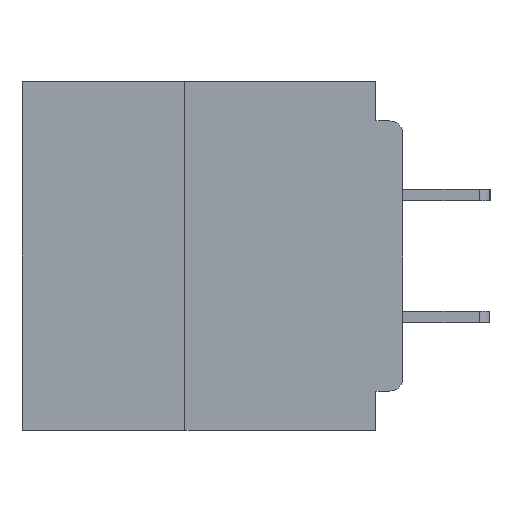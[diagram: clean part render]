
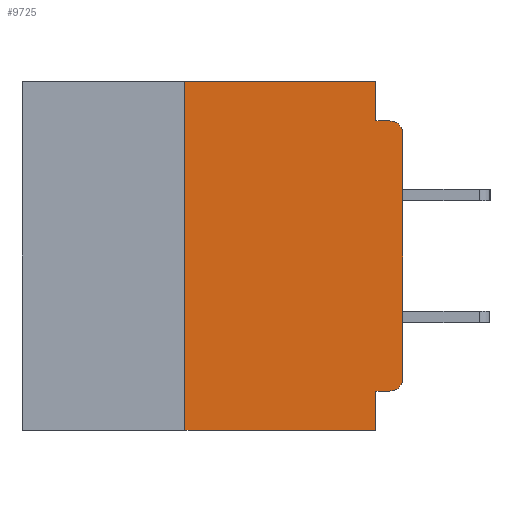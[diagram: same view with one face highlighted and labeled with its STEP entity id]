
A CAD part, left-side view. The second image highlights one B-rep face of the part: STEP entity #9725.
In plain terms, the highlighted planar face has unit normal (-1, 0, 0).
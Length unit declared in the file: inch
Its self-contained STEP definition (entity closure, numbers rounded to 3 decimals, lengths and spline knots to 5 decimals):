
#355 = EDGE_CURVE ( 'NONE', #34685, #10044, #22795, .T. ) ;
#2576 = DIRECTION ( 'NONE',  ( 0., 1., 0. ) ) ;
#2628 = CARTESIAN_POINT ( 'NONE',  ( 0., 0., -0.045 ) ) ;
#3607 = EDGE_CURVE ( 'NONE', #11408, #34685, #57170, .T. ) ;
#4150 = VECTOR ( 'NONE', #14899, 39.37008 ) ;
#4229 = ORIENTED_EDGE ( 'NONE', *, *, #5340, .T. ) ;
#5340 = EDGE_CURVE ( 'NONE', #44984, #27405, #8590, .T. ) ;
#5851 = CARTESIAN_POINT ( 'NONE',  ( 0., 0.015, -0.355 ) ) ;
#6154 = VERTEX_POINT ( 'NONE', #36166 ) ;
#6261 = DIRECTION ( 'NONE',  ( 0., 0., -1. ) ) ;
#7355 = CARTESIAN_POINT ( 'NONE',  ( 0., 0., -0.355 ) ) ;
#8275 = ORIENTED_EDGE ( 'NONE', *, *, #13251, .F. ) ;
#8430 = DIRECTION ( 'NONE',  ( 0., -1., 0. ) ) ;
#8469 = LINE ( 'NONE', #20610, #16781 ) ;
#8590 = CIRCLE ( 'NONE', #56082, 0.015 ) ;
#8843 = VECTOR ( 'NONE', #50147, 39.37008 ) ;
#9207 = CARTESIAN_POINT ( 'NONE',  ( 0., 0., -0.34 ) ) ;
#9725 = ADVANCED_FACE ( 'NONE', ( #29305 ), #10166, .F. ) ;
#10044 = VERTEX_POINT ( 'NONE', #59642 ) ;
#10106 = VECTOR ( 'NONE', #21964, 39.37008 ) ;
#10166 = PLANE ( 'NONE',  #30846 ) ;
#11242 = VECTOR ( 'NONE', #8430, 39.37008 ) ;
#11408 = VERTEX_POINT ( 'NONE', #30174 ) ;
#13251 = EDGE_CURVE ( 'NONE', #10044, #35344, #29674, .T. ) ;
#14317 = VERTEX_POINT ( 'NONE', #51814 ) ;
#14678 = CARTESIAN_POINT ( 'NONE',  ( 0., 0.031, 0. ) ) ;
#14899 = DIRECTION ( 'NONE',  ( 0., 0., -1. ) ) ;
#14999 = DIRECTION ( 'NONE',  ( 1., 0., 0. ) ) ;
#15138 = DIRECTION ( 'NONE',  ( 0., 0., 1. ) ) ;
#15150 = CARTESIAN_POINT ( 'NONE',  ( 0., 0.015, -0.34 ) ) ;
#16781 = VECTOR ( 'NONE', #6261, 39.37008 ) ;
#16835 = CARTESIAN_POINT ( 'NONE',  ( 0., 0., 0. ) ) ;
#19992 = DIRECTION ( 'NONE',  ( 0., 0., -1. ) ) ;
#20610 = CARTESIAN_POINT ( 'NONE',  ( 0., 0.031, -0.4 ) ) ;
#21021 = EDGE_LOOP ( 'NONE', ( #36286, #33792, #27893, #8275, #24023, #51731, #26784, #49543, #55724, #4229 ) ) ;
#21130 = EDGE_CURVE ( 'NONE', #27405, #31824, #58035, .T. ) ;
#21964 = DIRECTION ( 'NONE',  ( 0., -1., 0. ) ) ;
#22333 = EDGE_CURVE ( 'NONE', #35344, #6154, #48162, .T. ) ;
#22795 = LINE ( 'NONE', #52592, #59148 ) ;
#24023 = ORIENTED_EDGE ( 'NONE', *, *, #355, .F. ) ;
#24990 = DIRECTION ( 'NONE',  ( -1., 0., 0. ) ) ;
#26784 = ORIENTED_EDGE ( 'NONE', *, *, #59083, .T. ) ;
#27405 = VERTEX_POINT ( 'NONE', #9207 ) ;
#27893 = ORIENTED_EDGE ( 'NONE', *, *, #22333, .F. ) ;
#29305 = FACE_OUTER_BOUND ( 'NONE', #21021, .T. ) ;
#29375 = CARTESIAN_POINT ( 'NONE',  ( 0., 0.25, -0.4 ) ) ;
#29674 = LINE ( 'NONE', #14678, #4150 ) ;
#30174 = CARTESIAN_POINT ( 'NONE',  ( 0., 0.25, -0.4 ) ) ;
#30846 = AXIS2_PLACEMENT_3D ( 'NONE', #57613, #14999, #48334 ) ;
#31595 = VERTEX_POINT ( 'NONE', #48591 ) ;
#31824 = VERTEX_POINT ( 'NONE', #40895 ) ;
#33792 = ORIENTED_EDGE ( 'NONE', *, *, #50182, .T. ) ;
#34685 = VERTEX_POINT ( 'NONE', #57135 ) ;
#35344 = VERTEX_POINT ( 'NONE', #57264 ) ;
#36166 = CARTESIAN_POINT ( 'NONE',  ( 0., 0.015, -0.045 ) ) ;
#36263 = EDGE_CURVE ( 'NONE', #44984, #14317, #58942, .T. ) ;
#36286 = ORIENTED_EDGE ( 'NONE', *, *, #21130, .T. ) ;
#37107 = CARTESIAN_POINT ( 'NONE',  ( 0., 0.437, -0.4 ) ) ;
#40895 = CARTESIAN_POINT ( 'NONE',  ( 0., 0., -0.06 ) ) ;
#43122 = VECTOR ( 'NONE', #15138, 39.37008 ) ;
#43261 = EDGE_CURVE ( 'NONE', #14317, #31595, #8469, .T. ) ;
#44984 = VERTEX_POINT ( 'NONE', #5851 ) ;
#46382 = VECTOR ( 'NONE', #2576, 39.37008 ) ;
#48162 = LINE ( 'NONE', #2628, #10106 ) ;
#48334 = DIRECTION ( 'NONE',  ( 0., 0., -1. ) ) ;
#48489 = DIRECTION ( 'NONE',  ( -1., 0., 0. ) ) ;
#48591 = CARTESIAN_POINT ( 'NONE',  ( 0., 0.031, -0.4 ) ) ;
#49543 = ORIENTED_EDGE ( 'NONE', *, *, #43261, .F. ) ;
#50147 = DIRECTION ( 'NONE',  ( 0., 0., 1. ) ) ;
#50182 = EDGE_CURVE ( 'NONE', #31824, #6154, #54491, .T. ) ;
#51731 = ORIENTED_EDGE ( 'NONE', *, *, #3607, .F. ) ;
#51814 = CARTESIAN_POINT ( 'NONE',  ( 0., 0.031, -0.355 ) ) ;
#52592 = CARTESIAN_POINT ( 'NONE',  ( 0., 0.437, 0. ) ) ;
#52729 = DIRECTION ( 'NONE',  ( 0., -1., 0. ) ) ;
#53112 = AXIS2_PLACEMENT_3D ( 'NONE', #53414, #24990, #58158 ) ;
#53414 = CARTESIAN_POINT ( 'NONE',  ( 0., 0.015, -0.06 ) ) ;
#54491 = CIRCLE ( 'NONE', #53112, 0.015 ) ;
#55724 = ORIENTED_EDGE ( 'NONE', *, *, #36263, .F. ) ;
#56082 = AXIS2_PLACEMENT_3D ( 'NONE', #15150, #48489, #19992 ) ;
#57135 = CARTESIAN_POINT ( 'NONE',  ( 0., 0.25, 0. ) ) ;
#57170 = LINE ( 'NONE', #29375, #43122 ) ;
#57264 = CARTESIAN_POINT ( 'NONE',  ( 0., 0.031, -0.045 ) ) ;
#57613 = CARTESIAN_POINT ( 'NONE',  ( 0., 0.437, 0. ) ) ;
#58035 = LINE ( 'NONE', #16835, #8843 ) ;
#58158 = DIRECTION ( 'NONE',  ( 0., 0., -1. ) ) ;
#58942 = LINE ( 'NONE', #7355, #46382 ) ;
#59083 = EDGE_CURVE ( 'NONE', #11408, #31595, #60363, .T. ) ;
#59148 = VECTOR ( 'NONE', #52729, 39.37008 ) ;
#59642 = CARTESIAN_POINT ( 'NONE',  ( 0., 0.031, 0. ) ) ;
#60363 = LINE ( 'NONE', #37107, #11242 ) ;
